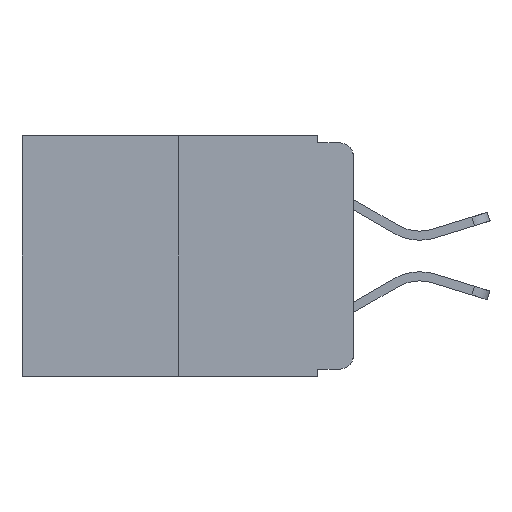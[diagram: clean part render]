
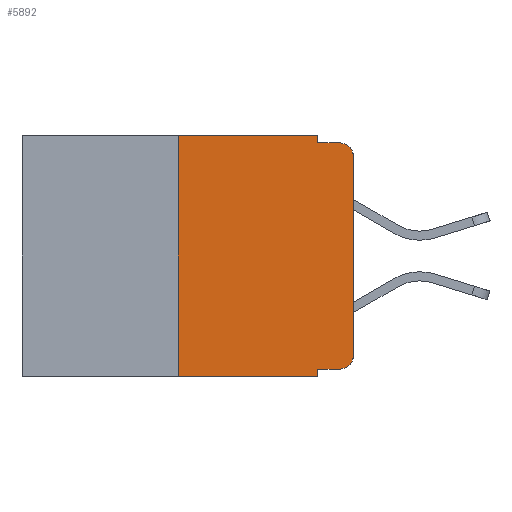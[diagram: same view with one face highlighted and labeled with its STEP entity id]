
A CAD part, left-side view. The second image highlights one B-rep face of the part: STEP entity #5892.
In plain terms, the highlighted planar face has unit normal (-1, 0, 0).
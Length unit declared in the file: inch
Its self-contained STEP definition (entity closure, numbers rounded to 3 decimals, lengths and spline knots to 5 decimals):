
#282 = DIRECTION ( 'NONE',  ( -1., 0., 0. ) ) ;
#410 = VERTEX_POINT ( 'NONE', #6496 ) ;
#497 = ORIENTED_EDGE ( 'NONE', *, *, #10463, .T. ) ;
#805 = EDGE_CURVE ( 'NONE', #11160, #9845, #9964, .T. ) ;
#1112 = VECTOR ( 'NONE', #4091, 39.37008 ) ;
#1450 = LINE ( 'NONE', #3152, #1112 ) ;
#1630 = EDGE_CURVE ( 'NONE', #9918, #2789, #9772, .T. ) ;
#1820 = CIRCLE ( 'NONE', #11377, 0.02 ) ;
#2292 = DIRECTION ( 'NONE',  ( 1., 0., 0. ) ) ;
#2426 = DIRECTION ( 'NONE',  ( -1., 0., 0. ) ) ;
#2732 = FACE_OUTER_BOUND ( 'NONE', #5677, .T. ) ;
#2789 = VERTEX_POINT ( 'NONE', #3859 ) ;
#2810 = VERTEX_POINT ( 'NONE', #10903 ) ;
#2862 = ORIENTED_EDGE ( 'NONE', *, *, #6866, .F. ) ;
#2984 = VECTOR ( 'NONE', #4311, 39.37008 ) ;
#2985 = CARTESIAN_POINT ( 'NONE',  ( 0., 0.051, 0. ) ) ;
#3021 = CARTESIAN_POINT ( 'NONE',  ( 0., 0., -0.03 ) ) ;
#3040 = CIRCLE ( 'NONE', #8275, 0.02 ) ;
#3149 = ORIENTED_EDGE ( 'NONE', *, *, #805, .T. ) ;
#3152 = CARTESIAN_POINT ( 'NONE',  ( 0., 0.051, -0.01 ) ) ;
#3183 = CARTESIAN_POINT ( 'NONE',  ( 0., 0., 0. ) ) ;
#3294 = LINE ( 'NONE', #2985, #5826 ) ;
#3313 = CARTESIAN_POINT ( 'NONE',  ( 0., 0.02, -0.333 ) ) ;
#3351 = CARTESIAN_POINT ( 'NONE',  ( 0., 0.051, -0.343 ) ) ;
#3436 = VECTOR ( 'NONE', #5518, 39.37008 ) ;
#3467 = VECTOR ( 'NONE', #3698, 39.37008 ) ;
#3698 = DIRECTION ( 'NONE',  ( 0., -1., 0. ) ) ;
#3859 = CARTESIAN_POINT ( 'NONE',  ( 0., 0.051, 0. ) ) ;
#3922 = DIRECTION ( 'NONE',  ( 0., 0., -1. ) ) ;
#4091 = DIRECTION ( 'NONE',  ( 0., -1., 0. ) ) ;
#4133 = DIRECTION ( 'NONE',  ( 0., 0., 1. ) ) ;
#4174 = CARTESIAN_POINT ( 'NONE',  ( 0., 0.473, 0. ) ) ;
#4280 = CARTESIAN_POINT ( 'NONE',  ( 0., 0.25, -0.343 ) ) ;
#4309 = EDGE_CURVE ( 'NONE', #11150, #4899, #1820, .T. ) ;
#4311 = DIRECTION ( 'NONE',  ( 0., -1., 0. ) ) ;
#4335 = VECTOR ( 'NONE', #4133, 39.37008 ) ;
#4382 = CARTESIAN_POINT ( 'NONE',  ( 0., 0.25, 0. ) ) ;
#4571 = CARTESIAN_POINT ( 'NONE',  ( 0., 0.25, 0. ) ) ;
#4749 = ORIENTED_EDGE ( 'NONE', *, *, #8095, .F. ) ;
#4899 = VERTEX_POINT ( 'NONE', #8990 ) ;
#4942 = LINE ( 'NONE', #6317, #9566 ) ;
#5335 = DIRECTION ( 'NONE',  ( 0., 0., -1. ) ) ;
#5518 = DIRECTION ( 'NONE',  ( 0., 0., 1. ) ) ;
#5576 = EDGE_CURVE ( 'NONE', #11285, #11150, #11057, .T. ) ;
#5677 = EDGE_LOOP ( 'NONE', ( #497, #8554, #9106, #4749, #7285, #2862, #3149, #5974, #11031, #11549 ) ) ;
#5826 = VECTOR ( 'NONE', #3922, 39.37008 ) ;
#5892 = ADVANCED_FACE ( 'NONE', ( #2732 ), #7045, .F. ) ;
#5974 = ORIENTED_EDGE ( 'NONE', *, *, #6244, .F. ) ;
#6244 = EDGE_CURVE ( 'NONE', #11285, #9845, #3294, .T. ) ;
#6263 = VERTEX_POINT ( 'NONE', #3021 ) ;
#6301 = CARTESIAN_POINT ( 'NONE',  ( 0., 0.473, -0.343 ) ) ;
#6304 = CARTESIAN_POINT ( 'NONE',  ( 0., 0.02, -0.313 ) ) ;
#6317 = CARTESIAN_POINT ( 'NONE',  ( 0., 0.051, 0. ) ) ;
#6478 = CARTESIAN_POINT ( 'NONE',  ( 0., 0.051, -0.333 ) ) ;
#6496 = CARTESIAN_POINT ( 'NONE',  ( 0., 0.051, -0.01 ) ) ;
#6866 = EDGE_CURVE ( 'NONE', #11160, #9918, #8416, .T. ) ;
#7045 = PLANE ( 'NONE',  #11959 ) ;
#7241 = DIRECTION ( 'NONE',  ( 0., 0., -1. ) ) ;
#7285 = ORIENTED_EDGE ( 'NONE', *, *, #1630, .F. ) ;
#7382 = CARTESIAN_POINT ( 'NONE',  ( 0., 0.473, 0. ) ) ;
#8091 = CARTESIAN_POINT ( 'NONE',  ( 0., 0.02, -0.03 ) ) ;
#8095 = EDGE_CURVE ( 'NONE', #2789, #410, #4942, .T. ) ;
#8275 = AXIS2_PLACEMENT_3D ( 'NONE', #8091, #2426, #8971 ) ;
#8416 = LINE ( 'NONE', #4571, #3436 ) ;
#8554 = ORIENTED_EDGE ( 'NONE', *, *, #9855, .T. ) ;
#8680 = EDGE_CURVE ( 'NONE', #410, #2810, #1450, .T. ) ;
#8845 = DIRECTION ( 'NONE',  ( 0., 0., -1. ) ) ;
#8971 = DIRECTION ( 'NONE',  ( 0., 0., -1. ) ) ;
#8990 = CARTESIAN_POINT ( 'NONE',  ( 0., 0., -0.313 ) ) ;
#9106 = ORIENTED_EDGE ( 'NONE', *, *, #8680, .F. ) ;
#9566 = VECTOR ( 'NONE', #5335, 39.37008 ) ;
#9699 = VECTOR ( 'NONE', #10853, 39.37008 ) ;
#9772 = LINE ( 'NONE', #7382, #2984 ) ;
#9845 = VERTEX_POINT ( 'NONE', #3351 ) ;
#9855 = EDGE_CURVE ( 'NONE', #6263, #2810, #3040, .T. ) ;
#9918 = VERTEX_POINT ( 'NONE', #4382 ) ;
#9964 = LINE ( 'NONE', #6301, #9699 ) ;
#10463 = EDGE_CURVE ( 'NONE', #4899, #6263, #11818, .T. ) ;
#10853 = DIRECTION ( 'NONE',  ( 0., -1., 0. ) ) ;
#10903 = CARTESIAN_POINT ( 'NONE',  ( 0., 0.02, -0.01 ) ) ;
#11031 = ORIENTED_EDGE ( 'NONE', *, *, #5576, .T. ) ;
#11057 = LINE ( 'NONE', #6478, #3467 ) ;
#11150 = VERTEX_POINT ( 'NONE', #3313 ) ;
#11160 = VERTEX_POINT ( 'NONE', #4280 ) ;
#11285 = VERTEX_POINT ( 'NONE', #11632 ) ;
#11377 = AXIS2_PLACEMENT_3D ( 'NONE', #6304, #282, #7241 ) ;
#11549 = ORIENTED_EDGE ( 'NONE', *, *, #4309, .T. ) ;
#11632 = CARTESIAN_POINT ( 'NONE',  ( 0., 0.051, -0.333 ) ) ;
#11818 = LINE ( 'NONE', #3183, #4335 ) ;
#11959 = AXIS2_PLACEMENT_3D ( 'NONE', #4174, #2292, #8845 ) ;
